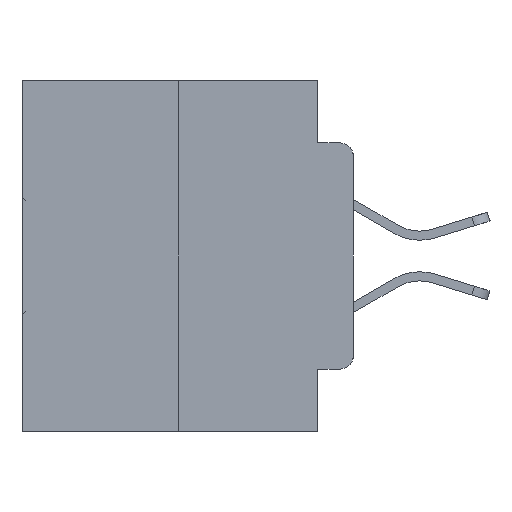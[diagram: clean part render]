
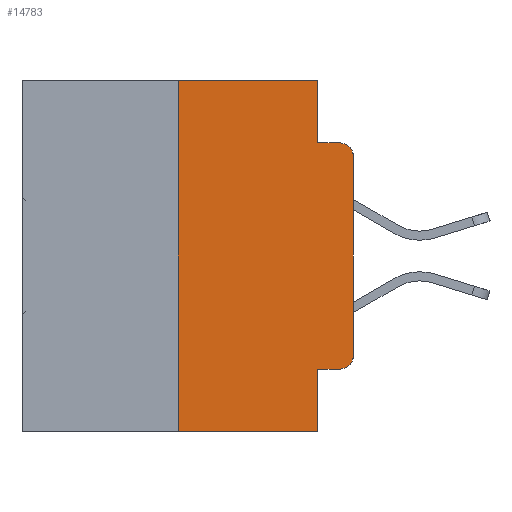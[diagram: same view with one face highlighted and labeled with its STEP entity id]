
A CAD part, left-side view. The second image highlights one B-rep face of the part: STEP entity #14783.
In plain terms, the highlighted planar face has unit normal (-1, 0, 0).
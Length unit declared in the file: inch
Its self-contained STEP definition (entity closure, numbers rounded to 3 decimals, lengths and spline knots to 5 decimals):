
#1188 = PLANE ( 'NONE',  #19968 ) ;
#2360 = VERTEX_POINT ( 'NONE', #17596 ) ;
#3135 = CARTESIAN_POINT ( 'NONE',  ( 0., 0., -0.3915 ) ) ;
#3657 = VECTOR ( 'NONE', #6434, 39.37008 ) ;
#3741 = DIRECTION ( 'NONE',  ( 1., 0., 0. ) ) ;
#3851 = VECTOR ( 'NONE', #28198, 39.37008 ) ;
#3906 = CARTESIAN_POINT ( 'NONE',  ( 0., 0.473, 0. ) ) ;
#4148 = VECTOR ( 'NONE', #12821, 39.37008 ) ;
#4493 = ORIENTED_EDGE ( 'NONE', *, *, #26538, .F. ) ;
#4554 = VECTOR ( 'NONE', #30289, 39.37008 ) ;
#4658 = EDGE_CURVE ( 'NONE', #5798, #14790, #11099, .T. ) ;
#4777 = DIRECTION ( 'NONE',  ( -1., 0., 0. ) ) ;
#4810 = LINE ( 'NONE', #25547, #16891 ) ;
#5217 = CARTESIAN_POINT ( 'NONE',  ( 0., 0.25, 0. ) ) ;
#5431 = LINE ( 'NONE', #13607, #11113 ) ;
#5569 = EDGE_LOOP ( 'NONE', ( #15785, #22792, #10910, #18759, #7502, #13901, #20950, #4493, #19167, #7927 ) ) ;
#5798 = VERTEX_POINT ( 'NONE', #19180 ) ;
#6161 = CARTESIAN_POINT ( 'NONE',  ( 0., 0.473, 0. ) ) ;
#6434 = DIRECTION ( 'NONE',  ( 0., -1., 0. ) ) ;
#7502 = ORIENTED_EDGE ( 'NONE', *, *, #9993, .F. ) ;
#7927 = ORIENTED_EDGE ( 'NONE', *, *, #28329, .T. ) ;
#8533 = DIRECTION ( 'NONE',  ( 0., 0., -1. ) ) ;
#9576 = VERTEX_POINT ( 'NONE', #21580 ) ;
#9993 = EDGE_CURVE ( 'NONE', #14790, #30504, #28212, .T. ) ;
#10372 = DIRECTION ( 'NONE',  ( -1., 0., 0. ) ) ;
#10910 = ORIENTED_EDGE ( 'NONE', *, *, #16008, .F. ) ;
#11099 = LINE ( 'NONE', #5217, #3851 ) ;
#11113 = VECTOR ( 'NONE', #27638, 39.37008 ) ;
#11146 = CARTESIAN_POINT ( 'NONE',  ( 0., 0.051, -0.0885 ) ) ;
#11380 = VERTEX_POINT ( 'NONE', #17209 ) ;
#11388 = LINE ( 'NONE', #19983, #4148 ) ;
#11786 = LINE ( 'NONE', #23481, #4554 ) ;
#12044 = CARTESIAN_POINT ( 'NONE',  ( 0., 0.051, 0. ) ) ;
#12789 = EDGE_CURVE ( 'NONE', #30504, #21117, #22435, .T. ) ;
#12821 = DIRECTION ( 'NONE',  ( 0., -1., 0. ) ) ;
#13607 = CARTESIAN_POINT ( 'NONE',  ( 0., 0.473, -0.5 ) ) ;
#13901 = ORIENTED_EDGE ( 'NONE', *, *, #4658, .F. ) ;
#14234 = CARTESIAN_POINT ( 'NONE',  ( 0., 0.051, -0.0885 ) ) ;
#14783 = ADVANCED_FACE ( 'NONE', ( #15638 ), #1188, .F. ) ;
#14790 = VERTEX_POINT ( 'NONE', #27976 ) ;
#15638 = FACE_OUTER_BOUND ( 'NONE', #5569, .T. ) ;
#15785 = ORIENTED_EDGE ( 'NONE', *, *, #28497, .T. ) ;
#15818 = VERTEX_POINT ( 'NONE', #3135 ) ;
#16008 = EDGE_CURVE ( 'NONE', #21117, #2360, #30503, .T. ) ;
#16891 = VECTOR ( 'NONE', #27859, 39.37008 ) ;
#17209 = CARTESIAN_POINT ( 'NONE',  ( 0., 0.051, -0.4115 ) ) ;
#17596 = CARTESIAN_POINT ( 'NONE',  ( 0., 0.02, -0.0885 ) ) ;
#18437 = CIRCLE ( 'NONE', #29808, 0.02 ) ;
#18759 = ORIENTED_EDGE ( 'NONE', *, *, #12789, .F. ) ;
#19167 = ORIENTED_EDGE ( 'NONE', *, *, #26765, .T. ) ;
#19180 = CARTESIAN_POINT ( 'NONE',  ( 0., 0.25, -0.5 ) ) ;
#19185 = CARTESIAN_POINT ( 'NONE',  ( 0., 0.02, -0.1085 ) ) ;
#19489 = EDGE_CURVE ( 'NONE', #5798, #30244, #5431, .T. ) ;
#19968 = AXIS2_PLACEMENT_3D ( 'NONE', #6161, #3741, #20567 ) ;
#19983 = CARTESIAN_POINT ( 'NONE',  ( 0., 0.051, -0.4115 ) ) ;
#20567 = DIRECTION ( 'NONE',  ( 0., 0., -1. ) ) ;
#20950 = ORIENTED_EDGE ( 'NONE', *, *, #19489, .T. ) ;
#21117 = VERTEX_POINT ( 'NONE', #14234 ) ;
#21515 = AXIS2_PLACEMENT_3D ( 'NONE', #24576, #10372, #26859 ) ;
#21536 = DIRECTION ( 'NONE',  ( 0., 0., -1. ) ) ;
#21580 = CARTESIAN_POINT ( 'NONE',  ( 0., 0.02, -0.4115 ) ) ;
#22315 = EDGE_CURVE ( 'NONE', #24774, #2360, #18437, .T. ) ;
#22435 = LINE ( 'NONE', #22791, #29987 ) ;
#22791 = CARTESIAN_POINT ( 'NONE',  ( 0., 0.051, 0. ) ) ;
#22792 = ORIENTED_EDGE ( 'NONE', *, *, #22315, .T. ) ;
#23481 = CARTESIAN_POINT ( 'NONE',  ( 0., 0.051, 0. ) ) ;
#24256 = CARTESIAN_POINT ( 'NONE',  ( 0., 0., -0.1085 ) ) ;
#24423 = VECTOR ( 'NONE', #27591, 39.37008 ) ;
#24576 = CARTESIAN_POINT ( 'NONE',  ( 0., 0.02, -0.3915 ) ) ;
#24774 = VERTEX_POINT ( 'NONE', #24256 ) ;
#25547 = CARTESIAN_POINT ( 'NONE',  ( 0., 0., 0. ) ) ;
#26538 = EDGE_CURVE ( 'NONE', #11380, #30244, #11786, .T. ) ;
#26765 = EDGE_CURVE ( 'NONE', #11380, #9576, #11388, .T. ) ;
#26859 = DIRECTION ( 'NONE',  ( 0., 0., -1. ) ) ;
#27454 = CARTESIAN_POINT ( 'NONE',  ( 0., 0.051, -0.5 ) ) ;
#27591 = DIRECTION ( 'NONE',  ( 0., -1., 0. ) ) ;
#27638 = DIRECTION ( 'NONE',  ( 0., -1., 0. ) ) ;
#27859 = DIRECTION ( 'NONE',  ( 0., 0., 1. ) ) ;
#27976 = CARTESIAN_POINT ( 'NONE',  ( 0., 0.25, 0. ) ) ;
#28198 = DIRECTION ( 'NONE',  ( 0., 0., 1. ) ) ;
#28212 = LINE ( 'NONE', #3906, #3657 ) ;
#28329 = EDGE_CURVE ( 'NONE', #9576, #15818, #28903, .T. ) ;
#28497 = EDGE_CURVE ( 'NONE', #15818, #24774, #4810, .T. ) ;
#28903 = CIRCLE ( 'NONE', #21515, 0.02 ) ;
#29808 = AXIS2_PLACEMENT_3D ( 'NONE', #19185, #4777, #21536 ) ;
#29987 = VECTOR ( 'NONE', #8533, 39.37008 ) ;
#30244 = VERTEX_POINT ( 'NONE', #27454 ) ;
#30289 = DIRECTION ( 'NONE',  ( 0., 0., -1. ) ) ;
#30503 = LINE ( 'NONE', #11146, #24423 ) ;
#30504 = VERTEX_POINT ( 'NONE', #12044 ) ;
